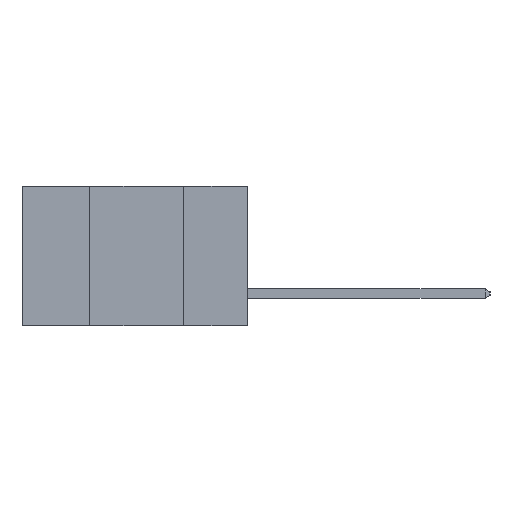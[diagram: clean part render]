
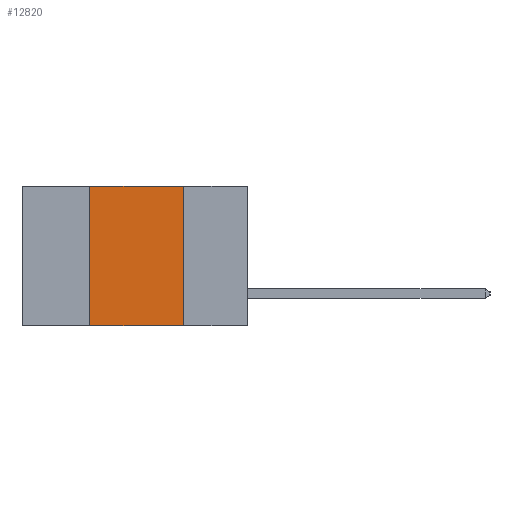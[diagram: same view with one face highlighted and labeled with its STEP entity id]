
A CAD part, left-side view. The second image highlights one B-rep face of the part: STEP entity #12820.
In plain terms, the highlighted planar face has unit normal (-1, 0, 0).
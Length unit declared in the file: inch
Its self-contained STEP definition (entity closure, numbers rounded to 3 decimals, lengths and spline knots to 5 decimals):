
#35 = CARTESIAN_POINT ( 'NONE',  ( 0., 0.6, 0. ) ) ;
#854 = VERTEX_POINT ( 'NONE', #10426 ) ;
#941 = LINE ( 'NONE', #35, #4958 ) ;
#1065 = LINE ( 'NONE', #7100, #7751 ) ;
#1074 = EDGE_CURVE ( 'NONE', #854, #11132, #2171, .T. ) ;
#1844 = VECTOR ( 'NONE', #16558, 39.37008 ) ;
#2171 = LINE ( 'NONE', #15082, #9210 ) ;
#2274 = PLANE ( 'NONE',  #15296 ) ;
#4812 = CARTESIAN_POINT ( 'NONE',  ( 0., 0.42, 0. ) ) ;
#4886 = EDGE_CURVE ( 'NONE', #854, #9921, #1065, .T. ) ;
#4958 = VECTOR ( 'NONE', #10653, 39.37008 ) ;
#4963 = DIRECTION ( 'NONE',  ( 0., 0., -1. ) ) ;
#5752 = ORIENTED_EDGE ( 'NONE', *, *, #4886, .T. ) ;
#6245 = CARTESIAN_POINT ( 'NONE',  ( 0., 0.17, 0. ) ) ;
#6798 = DIRECTION ( 'NONE',  ( 0., -1., 0. ) ) ;
#6839 = ORIENTED_EDGE ( 'NONE', *, *, #7675, .F. ) ;
#7100 = CARTESIAN_POINT ( 'NONE',  ( 0., 0.6, -0.37 ) ) ;
#7278 = EDGE_LOOP ( 'NONE', ( #6839, #7461, #9162, #5752 ) ) ;
#7461 = ORIENTED_EDGE ( 'NONE', *, *, #13712, .F. ) ;
#7555 = DIRECTION ( 'NONE',  ( 1., 0., 0. ) ) ;
#7675 = EDGE_CURVE ( 'NONE', #16710, #9921, #9304, .T. ) ;
#7751 = VECTOR ( 'NONE', #6798, 39.37008 ) ;
#9162 = ORIENTED_EDGE ( 'NONE', *, *, #1074, .F. ) ;
#9210 = VECTOR ( 'NONE', #10192, 39.37008 ) ;
#9304 = LINE ( 'NONE', #14018, #1844 ) ;
#9921 = VERTEX_POINT ( 'NONE', #10287 ) ;
#10192 = DIRECTION ( 'NONE',  ( 0., 0., 1. ) ) ;
#10287 = CARTESIAN_POINT ( 'NONE',  ( 0., 0.17, -0.37 ) ) ;
#10426 = CARTESIAN_POINT ( 'NONE',  ( 0., 0.42, -0.37 ) ) ;
#10653 = DIRECTION ( 'NONE',  ( 0., -1., 0. ) ) ;
#11132 = VERTEX_POINT ( 'NONE', #4812 ) ;
#12820 = ADVANCED_FACE ( 'NONE', ( #14491 ), #2274, .F. ) ;
#13712 = EDGE_CURVE ( 'NONE', #11132, #16710, #941, .T. ) ;
#14018 = CARTESIAN_POINT ( 'NONE',  ( 0., 0.17, -0.37 ) ) ;
#14491 = FACE_OUTER_BOUND ( 'NONE', #7278, .T. ) ;
#15082 = CARTESIAN_POINT ( 'NONE',  ( 0., 0.42, -0.37 ) ) ;
#15296 = AXIS2_PLACEMENT_3D ( 'NONE', #16489, #7555, #4963 ) ;
#16489 = CARTESIAN_POINT ( 'NONE',  ( 0., 0.6, 0. ) ) ;
#16558 = DIRECTION ( 'NONE',  ( 0., 0., -1. ) ) ;
#16710 = VERTEX_POINT ( 'NONE', #6245 ) ;
